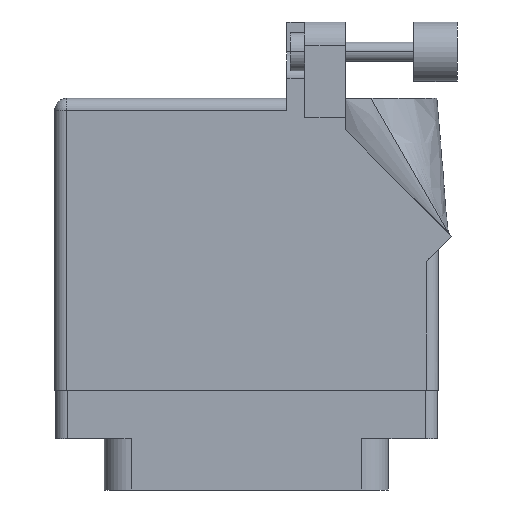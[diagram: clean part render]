
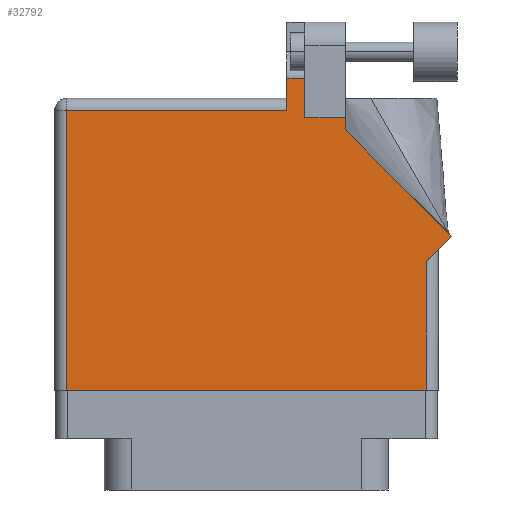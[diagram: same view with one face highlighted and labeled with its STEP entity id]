
A CAD part, front view. The second image highlights one B-rep face of the part: STEP entity #32792.
In plain terms, the highlighted face is planar.
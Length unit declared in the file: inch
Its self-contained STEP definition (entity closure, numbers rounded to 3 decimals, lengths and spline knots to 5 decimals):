
#1218 = FACE_OUTER_BOUND ( 'NONE', #3621, .T. ) ;
#1520 = EDGE_CURVE ( 'NONE', #32725, #7968, #8428, .T. ) ;
#1583 = CARTESIAN_POINT ( 'NONE',  ( 0.943, 0.637, 0.455 ) ) ;
#2403 = VECTOR ( 'NONE', #26623, 39.37008 ) ;
#2418 = DIRECTION ( 'NONE',  ( 0., 0., -1. ) ) ;
#2865 = CARTESIAN_POINT ( 'NONE',  ( 0.212, 1.43, 0.455 ) ) ;
#2981 = ORIENTED_EDGE ( 'NONE', *, *, #1520, .T. ) ;
#3381 = LINE ( 'NONE', #1583, #2403 ) ;
#3462 = EDGE_CURVE ( 'NONE', #17980, #32491, #33050, .T. ) ;
#3621 = EDGE_LOOP ( 'NONE', ( #12387, #20935, #4662, #25455, #16894, #2981, #33188, #20230, #38663, #26822, #11987 ) ) ;
#3635 = DIRECTION ( 'NONE',  ( 0., -1., 0. ) ) ;
#4269 = VECTOR ( 'NONE', #33737, 39.37008 ) ;
#4662 = ORIENTED_EDGE ( 'NONE', *, *, #21376, .T. ) ;
#4793 = CARTESIAN_POINT ( 'NONE',  ( 0.519, 1.33, 0.455 ) ) ;
#5032 = EDGE_CURVE ( 'NONE', #34306, #24690, #22522, .T. ) ;
#5321 = DIRECTION ( 'NONE',  ( -1., 0., 0. ) ) ;
#6199 = VECTOR ( 'NONE', #17747, 39.37008 ) ;
#6268 = DIRECTION ( 'NONE',  ( -1., 0., 0. ) ) ;
#6498 = VERTEX_POINT ( 'NONE', #31811 ) ;
#6816 = EDGE_CURVE ( 'NONE', #38656, #34159, #16910, .T. ) ;
#7702 = EDGE_CURVE ( 'NONE', #32491, #32725, #13344, .T. ) ;
#7766 = DIRECTION ( 'NONE',  ( 1., 0., 0. ) ) ;
#7929 = CARTESIAN_POINT ( 'NONE',  ( -1.005, 1.368, 0.455 ) ) ;
#7968 = VERTEX_POINT ( 'NONE', #32078 ) ;
#8257 = VERTEX_POINT ( 'NONE', #20970 ) ;
#8428 = LINE ( 'NONE', #26377, #29846 ) ;
#8484 = EDGE_CURVE ( 'NONE', #6498, #34306, #39566, .T. ) ;
#8527 = VERTEX_POINT ( 'NONE', #37764 ) ;
#8698 = DIRECTION ( 'NONE',  ( -1., 0., 0. ) ) ;
#9770 = CARTESIAN_POINT ( 'NONE',  ( -0.943, -0.1, 0.455 ) ) ;
#11559 = PLANE ( 'NONE',  #40034 ) ;
#11987 = ORIENTED_EDGE ( 'NONE', *, *, #24972, .T. ) ;
#11995 = CARTESIAN_POINT ( 'NONE',  ( 1.07571, 0.70771, 0.455 ) ) ;
#12387 = ORIENTED_EDGE ( 'NONE', *, *, #8484, .T. ) ;
#13344 = LINE ( 'NONE', #9770, #24983 ) ;
#14288 = VECTOR ( 'NONE', #6268, 39.37008 ) ;
#14322 = DIRECTION ( 'NONE',  ( -1., 0., 0. ) ) ;
#15524 = CARTESIAN_POINT ( 'NONE',  ( 0.63677, 1.5315, 0.455 ) ) ;
#15559 = DIRECTION ( 'NONE',  ( 0., 1., 0. ) ) ;
#15824 = CARTESIAN_POINT ( 'NONE',  ( -0.943, 1.368, 0.455 ) ) ;
#16894 = ORIENTED_EDGE ( 'NONE', *, *, #7702, .T. ) ;
#16910 = LINE ( 'NONE', #23429, #6199 ) ;
#17317 = LINE ( 'NONE', #2865, #27079 ) ;
#17534 = CARTESIAN_POINT ( 'NONE',  ( -0.943, -0.1, 0.455 ) ) ;
#17747 = DIRECTION ( 'NONE',  ( 0.707, 0.707, 0. ) ) ;
#17980 = VERTEX_POINT ( 'NONE', #36659 ) ;
#18654 = EDGE_CURVE ( 'NONE', #7968, #38656, #3381, .T. ) ;
#19544 = VECTOR ( 'NONE', #23727, 39.37008 ) ;
#20230 = ORIENTED_EDGE ( 'NONE', *, *, #6816, .T. ) ;
#20917 = CARTESIAN_POINT ( 'NONE',  ( -1.005, 1.43, 0.455 ) ) ;
#20935 = ORIENTED_EDGE ( 'NONE', *, *, #5032, .T. ) ;
#20970 = CARTESIAN_POINT ( 'NONE',  ( 0.519, 1.26442, 0.455 ) ) ;
#21376 = EDGE_CURVE ( 'NONE', #24690, #17980, #17317, .T. ) ;
#21510 = DIRECTION ( 'NONE',  ( 0., -1., 0. ) ) ;
#21651 = CARTESIAN_POINT ( 'NONE',  ( 0.306, 1.33, 0.455 ) ) ;
#21915 = LINE ( 'NONE', #4793, #31679 ) ;
#22522 = LINE ( 'NONE', #15524, #14288 ) ;
#22918 = VECTOR ( 'NONE', #15559, 39.37008 ) ;
#23429 = CARTESIAN_POINT ( 'NONE',  ( 1.005, 0.637, 0.455 ) ) ;
#23727 = DIRECTION ( 'NONE',  ( 0., 1., 0. ) ) ;
#24690 = VERTEX_POINT ( 'NONE', #37530 ) ;
#24972 = EDGE_CURVE ( 'NONE', #8527, #6498, #21915, .T. ) ;
#24983 = VECTOR ( 'NONE', #3635, 39.37008 ) ;
#25455 = ORIENTED_EDGE ( 'NONE', *, *, #3462, .T. ) ;
#26377 = CARTESIAN_POINT ( 'NONE',  ( -1.005, -0.1, 0.455 ) ) ;
#26623 = DIRECTION ( 'NONE',  ( 0., 1., 0. ) ) ;
#26822 = ORIENTED_EDGE ( 'NONE', *, *, #39532, .T. ) ;
#27079 = VECTOR ( 'NONE', #21510, 39.37008 ) ;
#27252 = EDGE_CURVE ( 'NONE', #34159, #8257, #33449, .T. ) ;
#29652 = VECTOR ( 'NONE', #14322, 39.37008 ) ;
#29846 = VECTOR ( 'NONE', #7766, 39.37008 ) ;
#31679 = VECTOR ( 'NONE', #5321, 39.37008 ) ;
#31811 = CARTESIAN_POINT ( 'NONE',  ( 0.306, 1.33, 0.455 ) ) ;
#32078 = CARTESIAN_POINT ( 'NONE',  ( 0.943, -0.1, 0.455 ) ) ;
#32491 = VERTEX_POINT ( 'NONE', #15824 ) ;
#32725 = VERTEX_POINT ( 'NONE', #17534 ) ;
#32792 = ADVANCED_FACE ( 'NONE', ( #1218 ), #11559, .F. ) ;
#33050 = LINE ( 'NONE', #7929, #29652 ) ;
#33188 = ORIENTED_EDGE ( 'NONE', *, *, #18654, .T. ) ;
#33449 = LINE ( 'NONE', #11995, #4269 ) ;
#33737 = DIRECTION ( 'NONE',  ( -0.707, 0.707, 0. ) ) ;
#34159 = VERTEX_POINT ( 'NONE', #37119 ) ;
#34306 = VERTEX_POINT ( 'NONE', #34497 ) ;
#34497 = CARTESIAN_POINT ( 'NONE',  ( 0.306, 1.5315, 0.455 ) ) ;
#35141 = LINE ( 'NONE', #35997, #19544 ) ;
#35997 = CARTESIAN_POINT ( 'NONE',  ( 0.519, 1.26442, 0.455 ) ) ;
#36659 = CARTESIAN_POINT ( 'NONE',  ( 0.212, 1.368, 0.455 ) ) ;
#36940 = CARTESIAN_POINT ( 'NONE',  ( 0.943, 0.575, 0.455 ) ) ;
#37119 = CARTESIAN_POINT ( 'NONE',  ( 1.07571, 0.70771, 0.455 ) ) ;
#37530 = CARTESIAN_POINT ( 'NONE',  ( 0.212, 1.5315, 0.455 ) ) ;
#37764 = CARTESIAN_POINT ( 'NONE',  ( 0.519, 1.33, 0.455 ) ) ;
#38656 = VERTEX_POINT ( 'NONE', #36940 ) ;
#38663 = ORIENTED_EDGE ( 'NONE', *, *, #27252, .T. ) ;
#39532 = EDGE_CURVE ( 'NONE', #8257, #8527, #35141, .T. ) ;
#39566 = LINE ( 'NONE', #21651, #22918 ) ;
#40034 = AXIS2_PLACEMENT_3D ( 'NONE', #20917, #2418, #8698 ) ;
